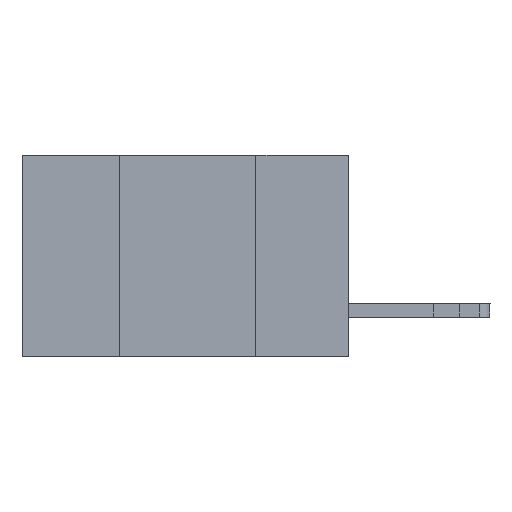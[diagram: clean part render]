
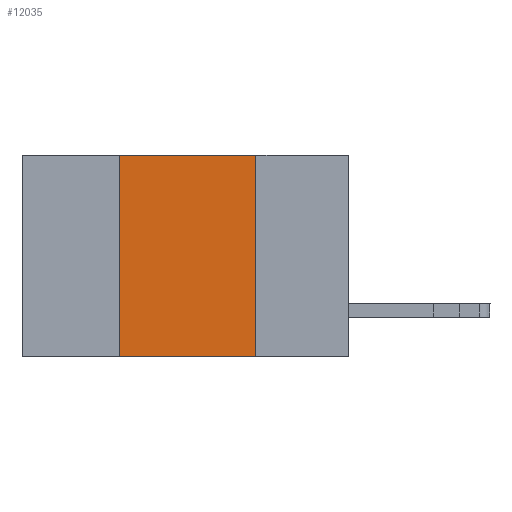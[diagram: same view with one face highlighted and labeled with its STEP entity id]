
A CAD part, left-side view. The second image highlights one B-rep face of the part: STEP entity #12035.
In plain terms, the highlighted planar face has unit normal (-1, 0, 0).
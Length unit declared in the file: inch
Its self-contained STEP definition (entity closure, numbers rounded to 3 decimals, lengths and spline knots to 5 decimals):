
#1362 = CARTESIAN_POINT ( 'NONE',  ( 0., 0.42, -0.37 ) ) ;
#1844 = DIRECTION ( 'NONE',  ( 0., -1., 0. ) ) ;
#2155 = LINE ( 'NONE', #15665, #12513 ) ;
#4255 = VECTOR ( 'NONE', #14974, 39.37008 ) ;
#4340 = VERTEX_POINT ( 'NONE', #12625 ) ;
#4468 = DIRECTION ( 'NONE',  ( 1., 0., 0. ) ) ;
#5151 = LINE ( 'NONE', #10062, #4255 ) ;
#5153 = CARTESIAN_POINT ( 'NONE',  ( 0., 0.42, 0. ) ) ;
#5327 = ORIENTED_EDGE ( 'NONE', *, *, #12852, .F. ) ;
#6183 = CARTESIAN_POINT ( 'NONE',  ( 0., 0.6, -0.37 ) ) ;
#6590 = ORIENTED_EDGE ( 'NONE', *, *, #15585, .F. ) ;
#7043 = VERTEX_POINT ( 'NONE', #1362 ) ;
#7049 = PLANE ( 'NONE',  #15804 ) ;
#7112 = EDGE_CURVE ( 'NONE', #7043, #12838, #7722, .T. ) ;
#7159 = EDGE_LOOP ( 'NONE', ( #5327, #6590, #7358, #11388 ) ) ;
#7358 = ORIENTED_EDGE ( 'NONE', *, *, #14186, .F. ) ;
#7587 = VERTEX_POINT ( 'NONE', #12839 ) ;
#7722 = LINE ( 'NONE', #6183, #13176 ) ;
#8691 = DIRECTION ( 'NONE',  ( 0., -1., 0. ) ) ;
#9314 = CARTESIAN_POINT ( 'NONE',  ( 0., 0.17, -0.37 ) ) ;
#10062 = CARTESIAN_POINT ( 'NONE',  ( 0., 0.17, 0. ) ) ;
#11279 = LINE ( 'NONE', #5153, #13556 ) ;
#11388 = ORIENTED_EDGE ( 'NONE', *, *, #7112, .T. ) ;
#11442 = DIRECTION ( 'NONE',  ( 0., 0., 1. ) ) ;
#12035 = ADVANCED_FACE ( 'NONE', ( #15488 ), #7049, .F. ) ;
#12513 = VECTOR ( 'NONE', #1844, 39.37008 ) ;
#12625 = CARTESIAN_POINT ( 'NONE',  ( 0., 0.42, 0. ) ) ;
#12838 = VERTEX_POINT ( 'NONE', #9314 ) ;
#12839 = CARTESIAN_POINT ( 'NONE',  ( 0., 0.17, 0. ) ) ;
#12852 = EDGE_CURVE ( 'NONE', #7587, #12838, #5151, .T. ) ;
#13157 = CARTESIAN_POINT ( 'NONE',  ( 0., 0.6, 0. ) ) ;
#13176 = VECTOR ( 'NONE', #8691, 39.37008 ) ;
#13556 = VECTOR ( 'NONE', #11442, 39.37008 ) ;
#14186 = EDGE_CURVE ( 'NONE', #7043, #4340, #11279, .T. ) ;
#14974 = DIRECTION ( 'NONE',  ( 0., 0., -1. ) ) ;
#15412 = DIRECTION ( 'NONE',  ( 0., 0., -1. ) ) ;
#15488 = FACE_OUTER_BOUND ( 'NONE', #7159, .T. ) ;
#15585 = EDGE_CURVE ( 'NONE', #4340, #7587, #2155, .T. ) ;
#15665 = CARTESIAN_POINT ( 'NONE',  ( 0., 0.6, 0. ) ) ;
#15804 = AXIS2_PLACEMENT_3D ( 'NONE', #13157, #4468, #15412 ) ;
